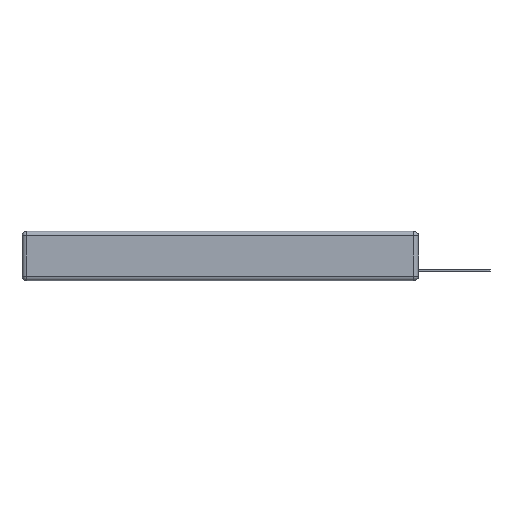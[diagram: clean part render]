
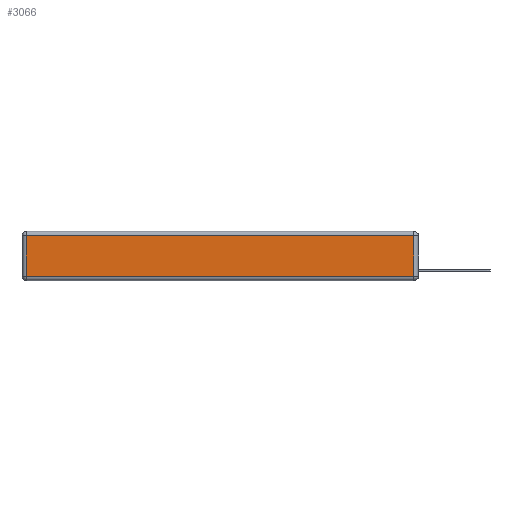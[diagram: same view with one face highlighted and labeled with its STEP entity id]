
A CAD part, left-side view. The second image highlights one B-rep face of the part: STEP entity #3066.
In plain terms, the highlighted planar face has unit normal (-1, 0, 0).
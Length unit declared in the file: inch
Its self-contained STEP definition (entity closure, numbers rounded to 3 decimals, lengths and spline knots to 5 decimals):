
#87 = CARTESIAN_POINT ( 'NONE',  ( 0., 0.03, -0.313 ) ) ;
#907 = VECTOR ( 'NONE', #6060, 39.37008 ) ;
#1016 = VERTEX_POINT ( 'NONE', #7581 ) ;
#1751 = VERTEX_POINT ( 'NONE', #87 ) ;
#3066 = ADVANCED_FACE ( 'NONE', ( #4378 ), #11300, .T. ) ;
#3121 = EDGE_CURVE ( 'NONE', #1751, #6208, #10578, .T. ) ;
#3135 = CARTESIAN_POINT ( 'NONE',  ( 0., 0., -0.343 ) ) ;
#3164 = LINE ( 'NONE', #12271, #6388 ) ;
#3699 = DIRECTION ( 'NONE',  ( 0., 0., -1. ) ) ;
#3760 = LINE ( 'NONE', #11941, #5935 ) ;
#4342 = ORIENTED_EDGE ( 'NONE', *, *, #11431, .T. ) ;
#4378 = FACE_OUTER_BOUND ( 'NONE', #11048, .T. ) ;
#4565 = CARTESIAN_POINT ( 'NONE',  ( 0., 0.03, -0.343 ) ) ;
#4666 = ORIENTED_EDGE ( 'NONE', *, *, #12672, .T. ) ;
#5613 = VECTOR ( 'NONE', #7625, 39.37008 ) ;
#5935 = VECTOR ( 'NONE', #3699, 39.37008 ) ;
#6060 = DIRECTION ( 'NONE',  ( 0., -1., 0. ) ) ;
#6208 = VERTEX_POINT ( 'NONE', #6728 ) ;
#6355 = ORIENTED_EDGE ( 'NONE', *, *, #3121, .T. ) ;
#6388 = VECTOR ( 'NONE', #11398, 39.37008 ) ;
#6587 = VERTEX_POINT ( 'NONE', #7643 ) ;
#6728 = CARTESIAN_POINT ( 'NONE',  ( 0., 0.03, -0.03 ) ) ;
#6933 = ORIENTED_EDGE ( 'NONE', *, *, #11525, .T. ) ;
#7062 = LINE ( 'NONE', #11073, #907 ) ;
#7581 = CARTESIAN_POINT ( 'NONE',  ( 0., 2.72, -0.313 ) ) ;
#7625 = DIRECTION ( 'NONE',  ( 0., 0., 1. ) ) ;
#7643 = CARTESIAN_POINT ( 'NONE',  ( 0., 2.72, -0.03 ) ) ;
#8410 = DIRECTION ( 'NONE',  ( 0., 0., 1. ) ) ;
#10313 = DIRECTION ( 'NONE',  ( -1., 0., 0. ) ) ;
#10578 = LINE ( 'NONE', #4565, #5613 ) ;
#11048 = EDGE_LOOP ( 'NONE', ( #6933, #6355, #4666, #4342 ) ) ;
#11073 = CARTESIAN_POINT ( 'NONE',  ( 0., 0., -0.313 ) ) ;
#11300 = PLANE ( 'NONE',  #12384 ) ;
#11398 = DIRECTION ( 'NONE',  ( 0., 1., 0. ) ) ;
#11431 = EDGE_CURVE ( 'NONE', #6587, #1016, #3760, .T. ) ;
#11525 = EDGE_CURVE ( 'NONE', #1016, #1751, #7062, .T. ) ;
#11941 = CARTESIAN_POINT ( 'NONE',  ( 0., 2.72, -0.343 ) ) ;
#12271 = CARTESIAN_POINT ( 'NONE',  ( 0., 2.75, -0.03 ) ) ;
#12384 = AXIS2_PLACEMENT_3D ( 'NONE', #3135, #10313, #8410 ) ;
#12672 = EDGE_CURVE ( 'NONE', #6208, #6587, #3164, .T. ) ;
